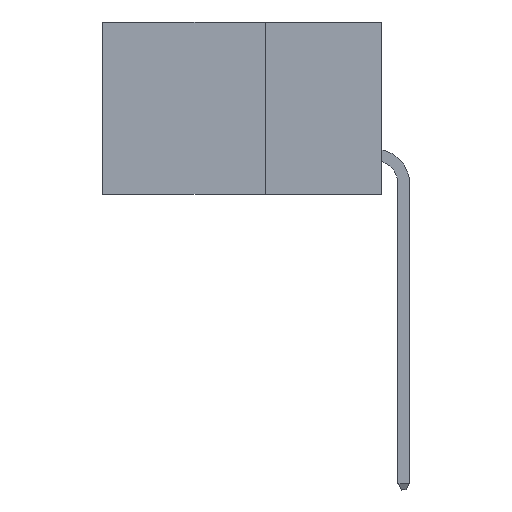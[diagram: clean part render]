
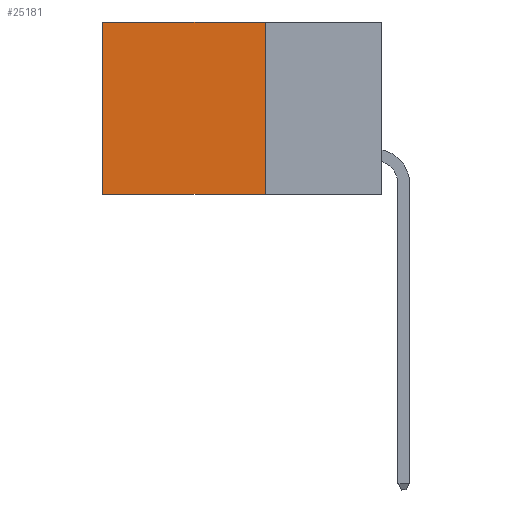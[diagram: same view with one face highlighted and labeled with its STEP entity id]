
A CAD part, left-side view. The second image highlights one B-rep face of the part: STEP entity #25181.
In plain terms, the highlighted planar face has unit normal (-1, 0, 0).
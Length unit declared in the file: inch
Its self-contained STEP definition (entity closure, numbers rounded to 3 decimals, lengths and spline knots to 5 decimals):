
#547 = DIRECTION ( 'NONE',  ( 0., 0., -1. ) ) ;
#786 = CARTESIAN_POINT ( 'NONE',  ( 0.2875, 0.6, 0. ) ) ;
#930 = CARTESIAN_POINT ( 'NONE',  ( 0.2875, 0.6, -0.37 ) ) ;
#1534 = FACE_OUTER_BOUND ( 'NONE', #10022, .T. ) ;
#1944 = CARTESIAN_POINT ( 'NONE',  ( 0.2875, 0.25, 0. ) ) ;
#3422 = ORIENTED_EDGE ( 'NONE', *, *, #3869, .T. ) ;
#3486 = PLANE ( 'NONE',  #28056 ) ;
#3869 = EDGE_CURVE ( 'NONE', #20730, #8856, #30605, .T. ) ;
#4407 = DIRECTION ( 'NONE',  ( 0., 0., -1. ) ) ;
#5070 = DIRECTION ( 'NONE',  ( 0., 1., 0. ) ) ;
#6281 = ORIENTED_EDGE ( 'NONE', *, *, #14306, .F. ) ;
#8755 = CARTESIAN_POINT ( 'NONE',  ( 0.2875, 0.25, -0.37 ) ) ;
#8856 = VERTEX_POINT ( 'NONE', #930 ) ;
#8945 = DIRECTION ( 'NONE',  ( 0., 1., 0. ) ) ;
#9410 = EDGE_CURVE ( 'NONE', #29625, #20730, #18200, .T. ) ;
#10022 = EDGE_LOOP ( 'NONE', ( #3422, #20696, #6281, #12333 ) ) ;
#12247 = VECTOR ( 'NONE', #547, 39.37008 ) ;
#12333 = ORIENTED_EDGE ( 'NONE', *, *, #9410, .T. ) ;
#12990 = LINE ( 'NONE', #27126, #12247 ) ;
#13153 = CARTESIAN_POINT ( 'NONE',  ( 0.2875, 0.25, 0. ) ) ;
#14306 = EDGE_CURVE ( 'NONE', #29625, #25072, #12990, .T. ) ;
#14341 = VECTOR ( 'NONE', #8945, 39.37008 ) ;
#15169 = CARTESIAN_POINT ( 'NONE',  ( 0.2875, 0.25, -0.37 ) ) ;
#15358 = DIRECTION ( 'NONE',  ( 0., 0., -1. ) ) ;
#15467 = CARTESIAN_POINT ( 'NONE',  ( 0.2875, 0.25, 0. ) ) ;
#15514 = VECTOR ( 'NONE', #4407, 39.37008 ) ;
#15737 = EDGE_CURVE ( 'NONE', #25072, #8856, #21529, .T. ) ;
#18200 = LINE ( 'NONE', #15467, #27223 ) ;
#20696 = ORIENTED_EDGE ( 'NONE', *, *, #15737, .F. ) ;
#20730 = VERTEX_POINT ( 'NONE', #786 ) ;
#21529 = LINE ( 'NONE', #8755, #14341 ) ;
#25072 = VERTEX_POINT ( 'NONE', #15169 ) ;
#25124 = CARTESIAN_POINT ( 'NONE',  ( 0.2875, 0.6, 0. ) ) ;
#25181 = ADVANCED_FACE ( 'NONE', ( #1534 ), #3486, .F. ) ;
#27126 = CARTESIAN_POINT ( 'NONE',  ( 0.2875, 0.25, 0. ) ) ;
#27223 = VECTOR ( 'NONE', #5070, 39.37008 ) ;
#28056 = AXIS2_PLACEMENT_3D ( 'NONE', #13153, #29901, #15358 ) ;
#29625 = VERTEX_POINT ( 'NONE', #1944 ) ;
#29901 = DIRECTION ( 'NONE',  ( 1., 0., 0. ) ) ;
#30605 = LINE ( 'NONE', #25124, #15514 ) ;
